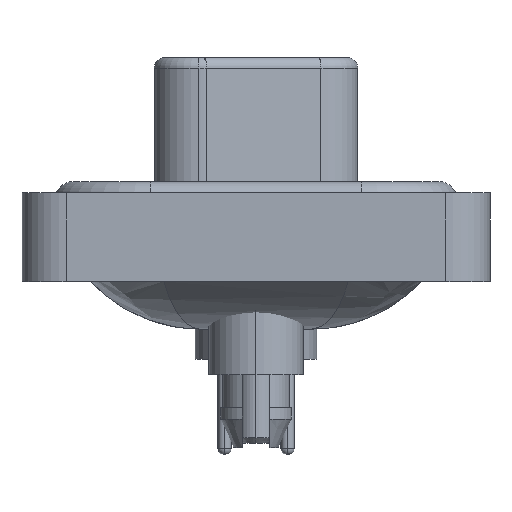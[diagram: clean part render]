
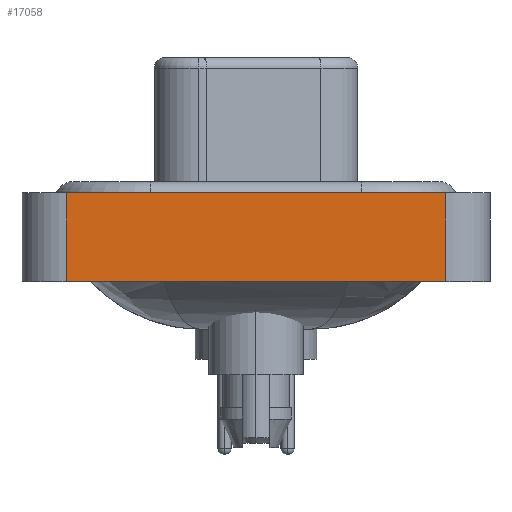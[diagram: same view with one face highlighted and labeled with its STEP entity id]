
A CAD part, left-side view. The second image highlights one B-rep face of the part: STEP entity #17058.
In plain terms, the highlighted planar face has unit normal (-1, 0, 0).
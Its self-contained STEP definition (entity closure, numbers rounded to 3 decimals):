
#639 = CARTESIAN_POINT ( 'NONE',  ( -7.35, -8.55, -3.6 ) ) ;
#1137 = CARTESIAN_POINT ( 'NONE',  ( -7.35, -8.55, 0.4 ) ) ;
#1162 = LINE ( 'NONE', #26058, #5039 ) ;
#2337 = LINE ( 'NONE', #25073, #6756 ) ;
#5039 = VECTOR ( 'NONE', #26202, 1000. ) ;
#5242 = LINE ( 'NONE', #639, #24817 ) ;
#6299 = PLANE ( 'NONE',  #23900 ) ;
#6339 = EDGE_CURVE ( 'NONE', #24184, #20385, #2337, .T. ) ;
#6402 = DIRECTION ( 'NONE',  ( 0., 0., 1. ) ) ;
#6756 = VECTOR ( 'NONE', #6402, 1000. ) ;
#8201 = DIRECTION ( 'NONE',  ( -1., 0., 0. ) ) ;
#8925 = DIRECTION ( 'NONE',  ( 0., -1., 0. ) ) ;
#10393 = FACE_OUTER_BOUND ( 'NONE', #23603, .T. ) ;
#10675 = VERTEX_POINT ( 'NONE', #20919 ) ;
#11488 = EDGE_CURVE ( 'NONE', #11497, #20385, #1162, .T. ) ;
#11497 = VERTEX_POINT ( 'NONE', #12427 ) ;
#12427 = CARTESIAN_POINT ( 'NONE',  ( -7.35, 8.55, 0.4 ) ) ;
#12515 = LINE ( 'NONE', #20807, #15623 ) ;
#14650 = EDGE_CURVE ( 'NONE', #10675, #11497, #12515, .T. ) ;
#14789 = ORIENTED_EDGE ( 'NONE', *, *, #11488, .F. ) ;
#15623 = VECTOR ( 'NONE', #20948, 1000. ) ;
#15788 = ORIENTED_EDGE ( 'NONE', *, *, #14650, .F. ) ;
#16243 = CARTESIAN_POINT ( 'NONE',  ( -7.35, -8.55, -3.6 ) ) ;
#17058 = ADVANCED_FACE ( 'NONE', ( #10393 ), #6299, .T. ) ;
#18299 = DIRECTION ( 'NONE',  ( 0., 0., 1. ) ) ;
#19993 = ORIENTED_EDGE ( 'NONE', *, *, #23092, .T. ) ;
#20385 = VERTEX_POINT ( 'NONE', #1137 ) ;
#20807 = CARTESIAN_POINT ( 'NONE',  ( -7.35, 8.55, -3.6 ) ) ;
#20919 = CARTESIAN_POINT ( 'NONE',  ( -7.35, 8.55, -3.6 ) ) ;
#20948 = DIRECTION ( 'NONE',  ( 0., 0., 1. ) ) ;
#22731 = ORIENTED_EDGE ( 'NONE', *, *, #6339, .T. ) ;
#23092 = EDGE_CURVE ( 'NONE', #10675, #24184, #5242, .T. ) ;
#23603 = EDGE_LOOP ( 'NONE', ( #22731, #14789, #15788, #19993 ) ) ;
#23900 = AXIS2_PLACEMENT_3D ( 'NONE', #16243, #8201, #18299 ) ;
#24184 = VERTEX_POINT ( 'NONE', #24887 ) ;
#24817 = VECTOR ( 'NONE', #8925, 1000. ) ;
#24887 = CARTESIAN_POINT ( 'NONE',  ( -7.35, -8.55, -3.6 ) ) ;
#25073 = CARTESIAN_POINT ( 'NONE',  ( -7.35, -8.55, -3.6 ) ) ;
#26058 = CARTESIAN_POINT ( 'NONE',  ( -7.35, -8.55, 0.4 ) ) ;
#26202 = DIRECTION ( 'NONE',  ( 0., -1., 0. ) ) ;
